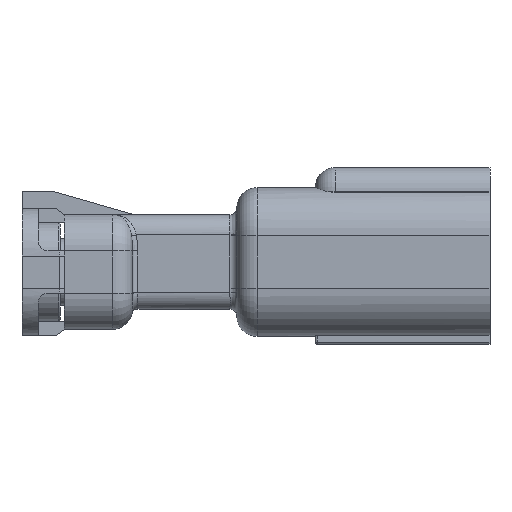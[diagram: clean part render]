
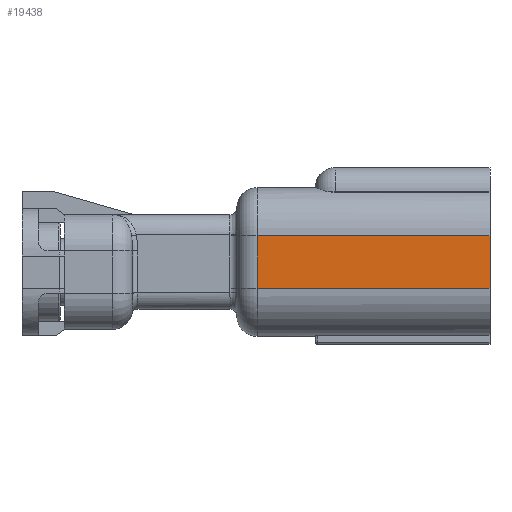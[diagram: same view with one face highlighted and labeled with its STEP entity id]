
A CAD part, left-side view. The second image highlights one B-rep face of the part: STEP entity #19438.
In plain terms, the highlighted planar face has unit normal (-1, 0, 0).
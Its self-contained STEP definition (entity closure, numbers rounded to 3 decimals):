
#1138 = CARTESIAN_POINT ( 'NONE',  ( -33.638, 22.336, 1.78 ) ) ;
#1353 = EDGE_CURVE ( 'NONE', #8701, #12849, #6701, .T. ) ;
#2065 = ORIENTED_EDGE ( 'NONE', *, *, #1353, .T. ) ;
#2532 = VECTOR ( 'NONE', #15098, 1000. ) ;
#2724 = VECTOR ( 'NONE', #20670, 1000. ) ;
#2987 = CARTESIAN_POINT ( 'NONE',  ( -33.638, 22.336, -3.22 ) ) ;
#4335 = DIRECTION ( 'NONE',  ( 0., -1., 0. ) ) ;
#5323 = EDGE_CURVE ( 'NONE', #12849, #11716, #13964, .T. ) ;
#5891 = ORIENTED_EDGE ( 'NONE', *, *, #5323, .T. ) ;
#6291 = LINE ( 'NONE', #13124, #20353 ) ;
#6644 = CARTESIAN_POINT ( 'NONE',  ( -33.638, 9.736, -3.22 ) ) ;
#6701 = LINE ( 'NONE', #1138, #7055 ) ;
#6786 = FACE_OUTER_BOUND ( 'NONE', #21859, .T. ) ;
#6787 = CARTESIAN_POINT ( 'NONE',  ( -33.638, 21.336, -0.82 ) ) ;
#7015 = DIRECTION ( 'NONE',  ( 1., 0., 0. ) ) ;
#7055 = VECTOR ( 'NONE', #17001, 1000. ) ;
#8300 = DIRECTION ( 'NONE',  ( 0., 0., -1. ) ) ;
#8375 = LINE ( 'NONE', #6644, #2532 ) ;
#8701 = VERTEX_POINT ( 'NONE', #12504 ) ;
#9232 = EDGE_CURVE ( 'NONE', #14181, #8701, #8375, .T. ) ;
#11716 = VERTEX_POINT ( 'NONE', #6787 ) ;
#11756 = AXIS2_PLACEMENT_3D ( 'NONE', #2987, #7015, #8300 ) ;
#12207 = ORIENTED_EDGE ( 'NONE', *, *, #21309, .T. ) ;
#12500 = CARTESIAN_POINT ( 'NONE',  ( -33.638, 9.736, -0.82 ) ) ;
#12504 = CARTESIAN_POINT ( 'NONE',  ( -33.638, 9.736, 1.78 ) ) ;
#12849 = VERTEX_POINT ( 'NONE', #22565 ) ;
#13124 = CARTESIAN_POINT ( 'NONE',  ( -33.638, 22.336, -0.82 ) ) ;
#13964 = LINE ( 'NONE', #14078, #2724 ) ;
#14078 = CARTESIAN_POINT ( 'NONE',  ( -33.638, 21.336, -0.82 ) ) ;
#14181 = VERTEX_POINT ( 'NONE', #12500 ) ;
#15098 = DIRECTION ( 'NONE',  ( 0., 0., 1. ) ) ;
#17001 = DIRECTION ( 'NONE',  ( 0., 1., 0. ) ) ;
#17428 = PLANE ( 'NONE',  #11756 ) ;
#19438 = ADVANCED_FACE ( 'NONE', ( #6786 ), #17428, .F. ) ;
#20353 = VECTOR ( 'NONE', #4335, 1000. ) ;
#20670 = DIRECTION ( 'NONE',  ( 0., 0., -1. ) ) ;
#21309 = EDGE_CURVE ( 'NONE', #11716, #14181, #6291, .T. ) ;
#21859 = EDGE_LOOP ( 'NONE', ( #2065, #5891, #12207, #21900 ) ) ;
#21900 = ORIENTED_EDGE ( 'NONE', *, *, #9232, .T. ) ;
#22565 = CARTESIAN_POINT ( 'NONE',  ( -33.638, 21.336, 1.78 ) ) ;
